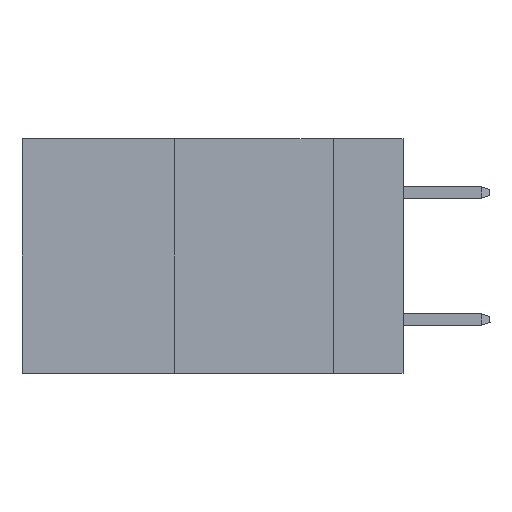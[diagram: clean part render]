
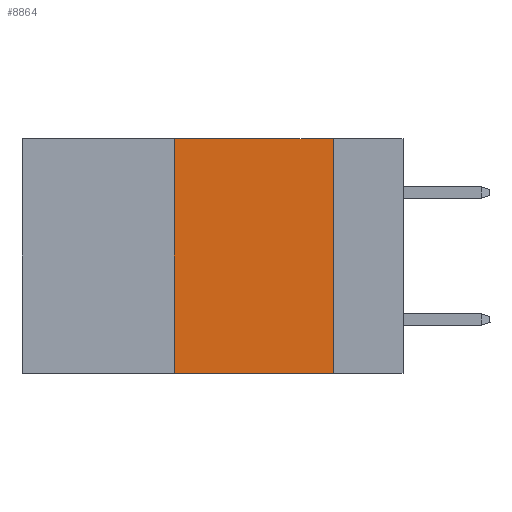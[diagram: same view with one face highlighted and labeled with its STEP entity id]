
A CAD part, left-side view. The second image highlights one B-rep face of the part: STEP entity #8864.
In plain terms, the highlighted planar face has unit normal (-1, 0, 0).
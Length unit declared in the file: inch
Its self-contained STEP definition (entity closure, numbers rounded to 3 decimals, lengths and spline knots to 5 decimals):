
#286 = LINE ( 'NONE', #13988, #554 ) ;
#554 = VECTOR ( 'NONE', #6465, 39.37008 ) ;
#990 = CARTESIAN_POINT ( 'NONE',  ( 0., 0.11, 0. ) ) ;
#1152 = LINE ( 'NONE', #6113, #13576 ) ;
#1242 = AXIS2_PLACEMENT_3D ( 'NONE', #2628, #7615, #4762 ) ;
#1422 = EDGE_CURVE ( 'NONE', #3947, #14257, #1467, .T. ) ;
#1467 = LINE ( 'NONE', #9130, #7543 ) ;
#2349 = EDGE_CURVE ( 'NONE', #14257, #5992, #286, .T. ) ;
#2460 = FACE_OUTER_BOUND ( 'NONE', #5300, .T. ) ;
#2628 = CARTESIAN_POINT ( 'NONE',  ( 0., 0.6, 0. ) ) ;
#2663 = EDGE_CURVE ( 'NONE', #3947, #7316, #1152, .T. ) ;
#2682 = DIRECTION ( 'NONE',  ( 0., 0., 1. ) ) ;
#3173 = ORIENTED_EDGE ( 'NONE', *, *, #1422, .F. ) ;
#3947 = VERTEX_POINT ( 'NONE', #5392 ) ;
#4015 = VECTOR ( 'NONE', #14960, 39.37008 ) ;
#4762 = DIRECTION ( 'NONE',  ( 0., 0., -1. ) ) ;
#5300 = EDGE_LOOP ( 'NONE', ( #6483, #11152, #3173, #10485 ) ) ;
#5392 = CARTESIAN_POINT ( 'NONE',  ( 0., 0.36, -0.37 ) ) ;
#5992 = VERTEX_POINT ( 'NONE', #990 ) ;
#6113 = CARTESIAN_POINT ( 'NONE',  ( 0., 0.6, -0.37 ) ) ;
#6465 = DIRECTION ( 'NONE',  ( 0., -1., 0. ) ) ;
#6483 = ORIENTED_EDGE ( 'NONE', *, *, #11760, .F. ) ;
#7316 = VERTEX_POINT ( 'NONE', #8342 ) ;
#7453 = PLANE ( 'NONE',  #1242 ) ;
#7543 = VECTOR ( 'NONE', #2682, 39.37008 ) ;
#7615 = DIRECTION ( 'NONE',  ( 1., 0., 0. ) ) ;
#8342 = CARTESIAN_POINT ( 'NONE',  ( 0., 0.11, -0.37 ) ) ;
#8864 = ADVANCED_FACE ( 'NONE', ( #2460 ), #7453, .F. ) ;
#9130 = CARTESIAN_POINT ( 'NONE',  ( 0., 0.36, 0. ) ) ;
#9640 = CARTESIAN_POINT ( 'NONE',  ( 0., 0.36, 0. ) ) ;
#9940 = CARTESIAN_POINT ( 'NONE',  ( 0., 0.11, 0. ) ) ;
#10485 = ORIENTED_EDGE ( 'NONE', *, *, #2663, .T. ) ;
#11119 = DIRECTION ( 'NONE',  ( 0., -1., 0. ) ) ;
#11152 = ORIENTED_EDGE ( 'NONE', *, *, #2349, .F. ) ;
#11760 = EDGE_CURVE ( 'NONE', #5992, #7316, #13872, .T. ) ;
#13576 = VECTOR ( 'NONE', #11119, 39.37008 ) ;
#13872 = LINE ( 'NONE', #9940, #4015 ) ;
#13988 = CARTESIAN_POINT ( 'NONE',  ( 0., 0.6, 0. ) ) ;
#14257 = VERTEX_POINT ( 'NONE', #9640 ) ;
#14960 = DIRECTION ( 'NONE',  ( 0., 0., -1. ) ) ;
